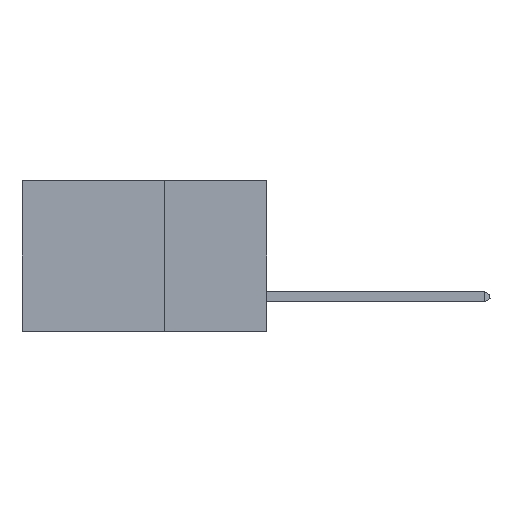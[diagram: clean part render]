
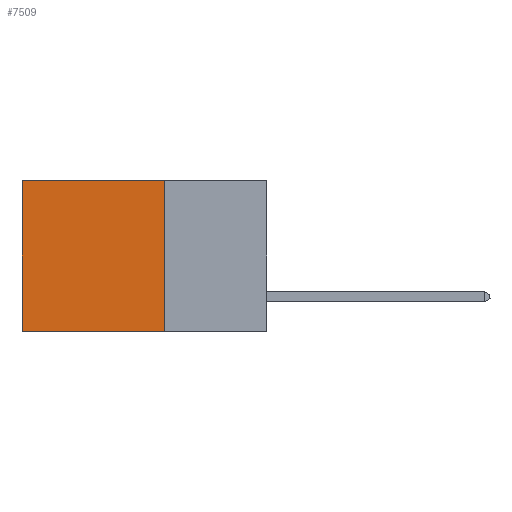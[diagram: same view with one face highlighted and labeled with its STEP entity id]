
A CAD part, left-side view. The second image highlights one B-rep face of the part: STEP entity #7509.
In plain terms, the highlighted planar face has unit normal (-1, 0, 0).
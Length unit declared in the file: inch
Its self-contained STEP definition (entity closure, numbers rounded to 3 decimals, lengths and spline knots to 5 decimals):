
#1411 = CARTESIAN_POINT ( 'NONE',  ( 0.2875, 0.25, 0. ) ) ;
#1677 = CARTESIAN_POINT ( 'NONE',  ( 0.2875, 0.6, 0. ) ) ;
#1852 = LINE ( 'NONE', #1411, #11043 ) ;
#1889 = ORIENTED_EDGE ( 'NONE', *, *, #8693, .F. ) ;
#2350 = VERTEX_POINT ( 'NONE', #13436 ) ;
#3601 = CARTESIAN_POINT ( 'NONE',  ( 0.2875, 0.6, 0. ) ) ;
#3714 = DIRECTION ( 'NONE',  ( 1., 0., 0. ) ) ;
#3783 = EDGE_CURVE ( 'NONE', #14357, #2350, #17321, .T. ) ;
#5985 = PLANE ( 'NONE',  #14169 ) ;
#6083 = FACE_OUTER_BOUND ( 'NONE', #12324, .T. ) ;
#7339 = DIRECTION ( 'NONE',  ( 0., 0., -1. ) ) ;
#7509 = ADVANCED_FACE ( 'NONE', ( #6083 ), #5985, .F. ) ;
#8693 = EDGE_CURVE ( 'NONE', #2350, #17240, #17172, .T. ) ;
#9325 = VECTOR ( 'NONE', #10494, 39.37008 ) ;
#9845 = EDGE_CURVE ( 'NONE', #14906, #17240, #13775, .T. ) ;
#10494 = DIRECTION ( 'NONE',  ( 0., 0., -1. ) ) ;
#10930 = DIRECTION ( 'NONE',  ( 0., 1., 0. ) ) ;
#11043 = VECTOR ( 'NONE', #10930, 39.37008 ) ;
#11442 = VECTOR ( 'NONE', #7339, 39.37008 ) ;
#11588 = ORIENTED_EDGE ( 'NONE', *, *, #9845, .T. ) ;
#12187 = CARTESIAN_POINT ( 'NONE',  ( 0.2875, 0.25, -0.37 ) ) ;
#12324 = EDGE_LOOP ( 'NONE', ( #11588, #1889, #17151, #12916 ) ) ;
#12626 = CARTESIAN_POINT ( 'NONE',  ( 0.2875, 0.25, 0. ) ) ;
#12916 = ORIENTED_EDGE ( 'NONE', *, *, #16933, .T. ) ;
#13436 = CARTESIAN_POINT ( 'NONE',  ( 0.2875, 0.25, -0.37 ) ) ;
#13614 = VECTOR ( 'NONE', #13902, 39.37008 ) ;
#13775 = LINE ( 'NONE', #3601, #9325 ) ;
#13902 = DIRECTION ( 'NONE',  ( 0., 1., 0. ) ) ;
#14169 = AXIS2_PLACEMENT_3D ( 'NONE', #16856, #3714, #17369 ) ;
#14357 = VERTEX_POINT ( 'NONE', #16355 ) ;
#14906 = VERTEX_POINT ( 'NONE', #1677 ) ;
#16243 = CARTESIAN_POINT ( 'NONE',  ( 0.2875, 0.6, -0.37 ) ) ;
#16355 = CARTESIAN_POINT ( 'NONE',  ( 0.2875, 0.25, 0. ) ) ;
#16856 = CARTESIAN_POINT ( 'NONE',  ( 0.2875, 0.25, 0. ) ) ;
#16933 = EDGE_CURVE ( 'NONE', #14357, #14906, #1852, .T. ) ;
#17151 = ORIENTED_EDGE ( 'NONE', *, *, #3783, .F. ) ;
#17172 = LINE ( 'NONE', #12187, #13614 ) ;
#17240 = VERTEX_POINT ( 'NONE', #16243 ) ;
#17321 = LINE ( 'NONE', #12626, #11442 ) ;
#17369 = DIRECTION ( 'NONE',  ( 0., 0., -1. ) ) ;
